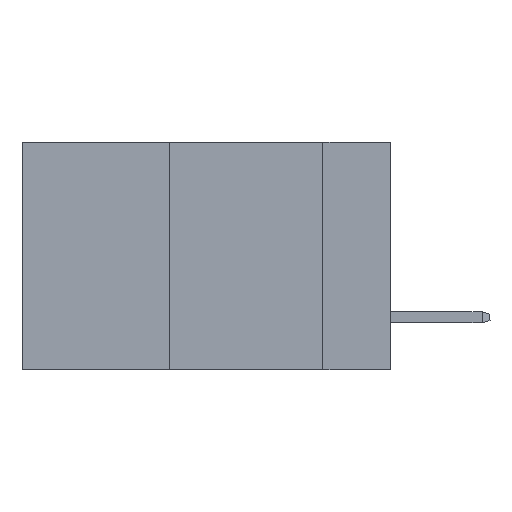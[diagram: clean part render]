
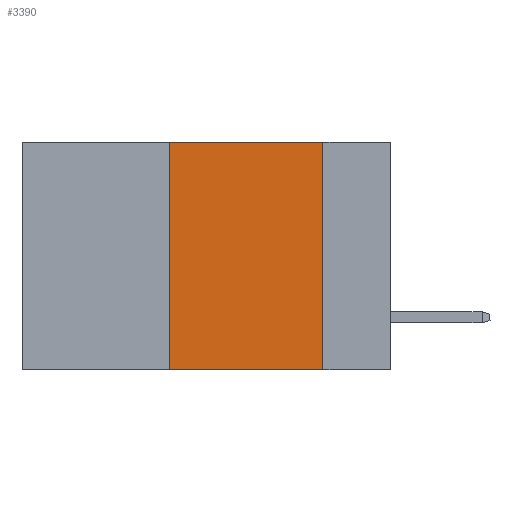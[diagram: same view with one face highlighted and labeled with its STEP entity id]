
A CAD part, left-side view. The second image highlights one B-rep face of the part: STEP entity #3390.
In plain terms, the highlighted planar face has unit normal (-1, 0, 0).
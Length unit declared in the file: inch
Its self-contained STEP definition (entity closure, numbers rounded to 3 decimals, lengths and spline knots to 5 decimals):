
#57 = VECTOR ( 'NONE', #4172, 39.37008 ) ;
#940 = ORIENTED_EDGE ( 'NONE', *, *, #3000, .F. ) ;
#1110 = FACE_OUTER_BOUND ( 'NONE', #6938, .T. ) ;
#2129 = VECTOR ( 'NONE', #7727, 39.37008 ) ;
#2523 = CARTESIAN_POINT ( 'NONE',  ( 0., 0.11, 0. ) ) ;
#2615 = DIRECTION ( 'NONE',  ( 0., 0., -1. ) ) ;
#2637 = EDGE_CURVE ( 'NONE', #5293, #4828, #10162, .T. ) ;
#2791 = EDGE_CURVE ( 'NONE', #5293, #8209, #8467, .T. ) ;
#3000 = EDGE_CURVE ( 'NONE', #8209, #4395, #6663, .T. ) ;
#3191 = CARTESIAN_POINT ( 'NONE',  ( 0., 0.11, -0.37 ) ) ;
#3390 = ADVANCED_FACE ( 'NONE', ( #1110 ), #10151, .F. ) ;
#3430 = LINE ( 'NONE', #3439, #7323 ) ;
#3439 = CARTESIAN_POINT ( 'NONE',  ( 0., 0.11, 0. ) ) ;
#3653 = CARTESIAN_POINT ( 'NONE',  ( 0., 0.36, 0. ) ) ;
#4172 = DIRECTION ( 'NONE',  ( 0., 0., 1. ) ) ;
#4247 = ORIENTED_EDGE ( 'NONE', *, *, #2791, .F. ) ;
#4395 = VERTEX_POINT ( 'NONE', #2523 ) ;
#4828 = VERTEX_POINT ( 'NONE', #3191 ) ;
#4933 = DIRECTION ( 'NONE',  ( 0., -1., 0. ) ) ;
#5090 = ORIENTED_EDGE ( 'NONE', *, *, #2637, .T. ) ;
#5197 = DIRECTION ( 'NONE',  ( 1., 0., 0. ) ) ;
#5293 = VERTEX_POINT ( 'NONE', #6986 ) ;
#5611 = CARTESIAN_POINT ( 'NONE',  ( 0., 0.36, 0. ) ) ;
#6005 = CARTESIAN_POINT ( 'NONE',  ( 0., 0.6, 0. ) ) ;
#6360 = AXIS2_PLACEMENT_3D ( 'NONE', #8993, #5197, #7158 ) ;
#6646 = ORIENTED_EDGE ( 'NONE', *, *, #7132, .F. ) ;
#6663 = LINE ( 'NONE', #6005, #8336 ) ;
#6938 = EDGE_LOOP ( 'NONE', ( #6646, #940, #4247, #5090 ) ) ;
#6986 = CARTESIAN_POINT ( 'NONE',  ( 0., 0.36, -0.37 ) ) ;
#7132 = EDGE_CURVE ( 'NONE', #4395, #4828, #3430, .T. ) ;
#7158 = DIRECTION ( 'NONE',  ( 0., 0., -1. ) ) ;
#7323 = VECTOR ( 'NONE', #2615, 39.37008 ) ;
#7727 = DIRECTION ( 'NONE',  ( 0., -1., 0. ) ) ;
#8209 = VERTEX_POINT ( 'NONE', #5611 ) ;
#8336 = VECTOR ( 'NONE', #4933, 39.37008 ) ;
#8467 = LINE ( 'NONE', #3653, #57 ) ;
#8567 = CARTESIAN_POINT ( 'NONE',  ( 0., 0.6, -0.37 ) ) ;
#8993 = CARTESIAN_POINT ( 'NONE',  ( 0., 0.6, 0. ) ) ;
#10151 = PLANE ( 'NONE',  #6360 ) ;
#10162 = LINE ( 'NONE', #8567, #2129 ) ;
